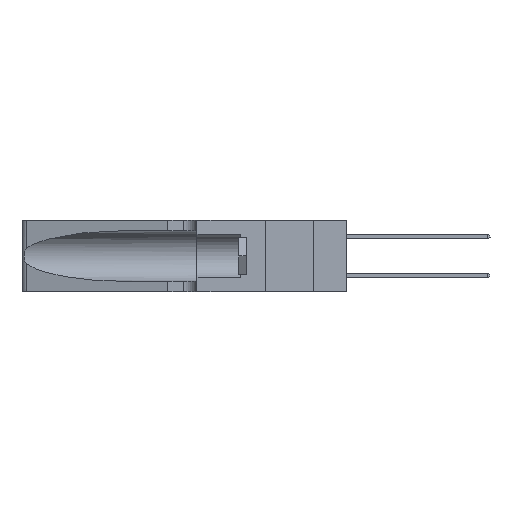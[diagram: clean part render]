
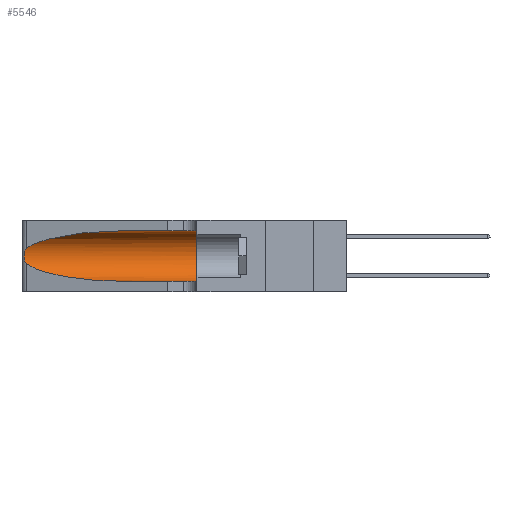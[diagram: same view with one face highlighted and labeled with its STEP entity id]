
A CAD part, left-side view. The second image highlights one B-rep face of the part: STEP entity #5546.
In plain terms, the highlighted cylindrical face has radius 3.308 mm (diameter 6.617 mm), a partial arc.
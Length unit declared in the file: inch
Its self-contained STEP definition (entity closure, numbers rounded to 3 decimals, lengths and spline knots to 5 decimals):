
#1 = CARTESIAN_POINT ( 'NONE',  ( 0.25487, 1.22718, 0.22369 ) ) ;
#894 = EDGE_CURVE ( 'NONE', #44993, #5187, #38678, .T. ) ;
#1451 = CARTESIAN_POINT ( 'NONE',  ( 0.1305, 0.35, 0.31525 ) ) ;
#2002 = CARTESIAN_POINT ( 'NONE',  ( 0.25789, 1.23486, 0.15765 ) ) ;
#2438 = VERTEX_POINT ( 'NONE', #22071 ) ;
#3133 = ORIENTED_EDGE ( 'NONE', *, *, #27404, .T. ) ;
#4183 = FACE_OUTER_BOUND ( 'NONE', #27237, .T. ) ;
#4443 = CARTESIAN_POINT ( 'NONE',  ( 0.18966, 0.96281, 0.31525 ) ) ;
#4917 = VECTOR ( 'NONE', #6272, 39.37008 ) ;
#5187 = VERTEX_POINT ( 'NONE', #12450 ) ;
#5418 = CARTESIAN_POINT ( 'NONE',  ( 0.25555, 1.22994, 0.2215 ) ) ;
#5546 = ADVANCED_FACE ( 'NONE', ( #4183 ), #12413, .F. ) ;
#5571 = CARTESIAN_POINT ( 'NONE',  ( 0.25555, 1.22993, 0.14849 ) ) ;
#5633 = EDGE_CURVE ( 'NONE', #5187, #2438, #22613, .T. ) ;
#6032 = LINE ( 'NONE', #30586, #4917 ) ;
#6272 = DIRECTION ( 'NONE',  ( 0., -1., 0. ) ) ;
#7619 = ORIENTED_EDGE ( 'NONE', *, *, #18518, .F. ) ;
#8149 = CARTESIAN_POINT ( 'NONE',  ( 0.25487, 1.22718, 0.22369 ) ) ;
#8951 = CARTESIAN_POINT ( 'NONE',  ( 0.25487, 1.22718, 0.22369 ) ) ;
#9265 = DIRECTION ( 'NONE',  ( 0., 0., -1. ) ) ;
#9718 = CARTESIAN_POINT ( 'NONE',  ( 0.25487, 1.22718, 0.14631 ) ) ;
#12411 = LINE ( 'NONE', #24657, #20574 ) ;
#12413 = CYLINDRICAL_SURFACE ( 'NONE', #33614, 0.13025 ) ;
#12450 = CARTESIAN_POINT ( 'NONE',  ( 0.25487, 1.22718, 0.14631 ) ) ;
#12471 = CARTESIAN_POINT ( 'NONE',  ( 0.25787, 1.23484, 0.2124 ) ) ;
#14354 = DIRECTION ( 'NONE',  ( 0., -1., 0. ) ) ;
#15008 = CARTESIAN_POINT ( 'NONE',  ( 0.1305, 0.72297, 0.31525 ) ) ;
#15964 = CARTESIAN_POINT ( 'NONE',  ( 0.26018, 1.23835, 0.19895 ) ) ;
#16490 = CARTESIAN_POINT ( 'NONE',  ( 0.1305, 0.35, 0.185 ) ) ;
#16718 = CARTESIAN_POINT ( 'NONE',  ( 0.1305, 0.72297, 0.05475 ) ) ;
#18518 = EDGE_CURVE ( 'NONE', #25641, #38203, #12411, .T. ) ;
#19029 = ORIENTED_EDGE ( 'NONE', *, *, #894, .T. ) ;
#19210 = CARTESIAN_POINT ( 'NONE',  ( 0.1305, 0.35, 0.05475 ) ) ;
#19473 = CARTESIAN_POINT ( 'NONE',  ( 0.26075, 1.23896, 0.178 ) ) ;
#19977 = DIRECTION ( 'NONE',  ( 0., 0., 1. ) ) ;
#20304 = EDGE_CURVE ( 'NONE', #38203, #30867, #21481, .T. ) ;
#20574 = VECTOR ( 'NONE', #14354, 39.37008 ) ;
#21481 = CIRCLE ( 'NONE', #22868, 0.13025 ) ;
#22071 = CARTESIAN_POINT ( 'NONE',  ( 0.1305, 0.72297, 0.05475 ) ) ;
#22613 =( BOUNDED_CURVE ( )  B_SPLINE_CURVE ( 3, ( #9718, #30501, #37394, #16718 ),
 .UNSPECIFIED., .F., .F. ) 
 B_SPLINE_CURVE_WITH_KNOTS ( ( 4, 4 ),
 ( 3.44316, 4.71239 ),
 .UNSPECIFIED. ) 
 CURVE ( )  GEOMETRIC_REPRESENTATION_ITEM ( )  RATIONAL_B_SPLINE_CURVE ( ( 1., 0.87, 0.87, 1. ) ) 
 REPRESENTATION_ITEM ( '' )  );
#22868 = AXIS2_PLACEMENT_3D ( 'NONE', #16490, #40667, #19977 ) ;
#22943 = CARTESIAN_POINT ( 'NONE',  ( 0.25856, 1.23593, 0.16098 ) ) ;
#23083 = CARTESIAN_POINT ( 'NONE',  ( 0.1305, 1.61858, 0.185 ) ) ;
#23380 = ORIENTED_EDGE ( 'NONE', *, *, #5633, .T. ) ;
#24657 = CARTESIAN_POINT ( 'NONE',  ( 0.1305, 1.61858, 0.31525 ) ) ;
#25010 = ORIENTED_EDGE ( 'NONE', *, *, #20304, .F. ) ;
#25641 = VERTEX_POINT ( 'NONE', #31575 ) ;
#26279 = CARTESIAN_POINT ( 'NONE',  ( 0.25639, 1.23184, 0.21858 ) ) ;
#26429 = CARTESIAN_POINT ( 'NONE',  ( 0.25639, 1.23186, 0.15144 ) ) ;
#27237 = EDGE_LOOP ( 'NONE', ( #3133, #19029, #23380, #44972, #25010, #7619 ) ) ;
#27404 = EDGE_CURVE ( 'NONE', #25641, #44993, #35350, .T. ) ;
#28942 = CARTESIAN_POINT ( 'NONE',  ( 0.2373, 1.15595, 0.28018 ) ) ;
#29899 = CARTESIAN_POINT ( 'NONE',  ( 0.25487, 1.22718, 0.14631 ) ) ;
#30052 = DIRECTION ( 'NONE',  ( 0., -1., 0. ) ) ;
#30501 = CARTESIAN_POINT ( 'NONE',  ( 0.2373, 1.15595, 0.08982 ) ) ;
#30586 = CARTESIAN_POINT ( 'NONE',  ( 0.1305, 1.61858, 0.05475 ) ) ;
#30867 = VERTEX_POINT ( 'NONE', #19210 ) ;
#31575 = CARTESIAN_POINT ( 'NONE',  ( 0.1305, 0.72297, 0.31525 ) ) ;
#32419 = EDGE_CURVE ( 'NONE', #2438, #30867, #6032, .T. ) ;
#33614 = AXIS2_PLACEMENT_3D ( 'NONE', #23083, #30052, #9265 ) ;
#35350 =( BOUNDED_CURVE ( )  B_SPLINE_CURVE ( 3, ( #15008, #4443, #28942, #8149 ),
 .UNSPECIFIED., .F., .T. ) 
 B_SPLINE_CURVE_WITH_KNOTS ( ( 4, 4 ),
 ( 1.5708, 2.84003 ),
 .UNSPECIFIED. ) 
 CURVE ( )  GEOMETRIC_REPRESENTATION_ITEM ( )  RATIONAL_B_SPLINE_CURVE ( ( 1., 0.87, 0.87, 1. ) ) 
 REPRESENTATION_ITEM ( '' )  );
#36653 = CARTESIAN_POINT ( 'NONE',  ( 0.25854, 1.2359, 0.20912 ) ) ;
#37394 = CARTESIAN_POINT ( 'NONE',  ( 0.18966, 0.96281, 0.05475 ) ) ;
#38203 = VERTEX_POINT ( 'NONE', #1451 ) ;
#38678 = B_SPLINE_CURVE_WITH_KNOTS ( 'NONE', 3,
 ( #8951, #5418, #26279, #12471, #36653, #15964, #40143, #19473, #43615, #22943, #2002, #26429, #5571, #29899 ),
 .UNSPECIFIED., .F., .F.,
 ( 4, 2, 2, 2, 2, 2, 4 ),
 ( 0., 0.00027, 0.00053, 0.00107, 0.0016, 0.00187, 0.00214 ),
 .UNSPECIFIED. ) ;
#40143 = CARTESIAN_POINT ( 'NONE',  ( 0.26075, 1.23896, 0.19203 ) ) ;
#40667 = DIRECTION ( 'NONE',  ( 0., 1., 0. ) ) ;
#43615 = CARTESIAN_POINT ( 'NONE',  ( 0.26017, 1.23833, 0.17102 ) ) ;
#44972 = ORIENTED_EDGE ( 'NONE', *, *, #32419, .T. ) ;
#44993 = VERTEX_POINT ( 'NONE', #1 ) ;
